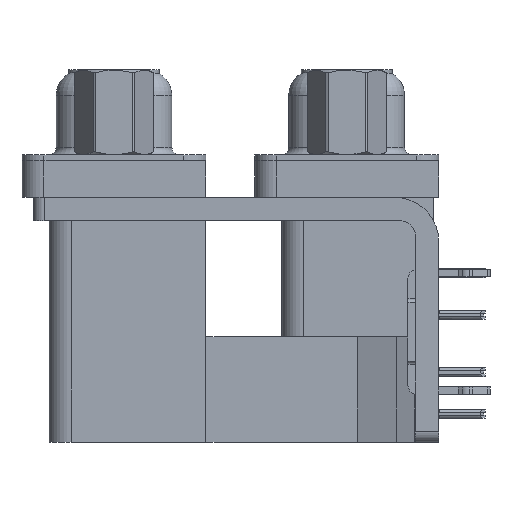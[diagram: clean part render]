
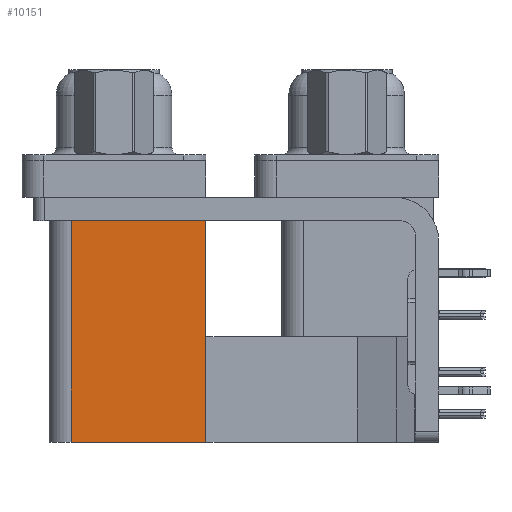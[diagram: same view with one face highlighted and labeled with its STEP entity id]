
A CAD part, left-side view. The second image highlights one B-rep face of the part: STEP entity #10151.
In plain terms, the highlighted planar face has unit normal (-1, 0, 0).
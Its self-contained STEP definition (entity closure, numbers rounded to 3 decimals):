
#3024 = EDGE_CURVE ( 'NONE', #4652, #26263, #17818, .T. ) ;
#3674 = AXIS2_PLACEMENT_3D ( 'NONE', #4900, #19683, #19929 ) ;
#4652 = VERTEX_POINT ( 'NONE', #45488 ) ;
#4900 = CARTESIAN_POINT ( 'NONE',  ( 3.79, 9.6, -19.2 ) ) ;
#7055 = DIRECTION ( 'NONE',  ( 0., 1., 0. ) ) ;
#7793 = CARTESIAN_POINT ( 'NONE',  ( 3.79, 18.8, -2.5 ) ) ;
#10151 = ADVANCED_FACE ( 'NONE', ( #31162 ), #35183, .F. ) ;
#10164 = VECTOR ( 'NONE', #33649, 1000. ) ;
#11570 = EDGE_CURVE ( 'NONE', #33424, #26263, #18388, .T. ) ;
#11729 = EDGE_CURVE ( 'NONE', #20270, #33424, #15848, .T. ) ;
#14652 = EDGE_CURVE ( 'NONE', #20270, #4652, #35381, .T. ) ;
#15076 = VECTOR ( 'NONE', #47637, 1000. ) ;
#15828 = ORIENTED_EDGE ( 'NONE', *, *, #14652, .T. ) ;
#15848 = LINE ( 'NONE', #42152, #46941 ) ;
#17818 = LINE ( 'NONE', #41332, #23950 ) ;
#18388 = LINE ( 'NONE', #41407, #10164 ) ;
#19683 = DIRECTION ( 'NONE',  ( 1., 0., 0. ) ) ;
#19929 = DIRECTION ( 'NONE',  ( 0., 1., 0. ) ) ;
#20270 = VERTEX_POINT ( 'NONE', #42374 ) ;
#23107 = ORIENTED_EDGE ( 'NONE', *, *, #11729, .F. ) ;
#23950 = VECTOR ( 'NONE', #7055, 1000. ) ;
#24110 = CARTESIAN_POINT ( 'NONE',  ( 3.79, 9.6, -19.2 ) ) ;
#24972 = ORIENTED_EDGE ( 'NONE', *, *, #11570, .F. ) ;
#26263 = VERTEX_POINT ( 'NONE', #7793 ) ;
#27074 = EDGE_LOOP ( 'NONE', ( #46487, #24972, #23107, #15828 ) ) ;
#30866 = CARTESIAN_POINT ( 'NONE',  ( 3.79, 18.8, -19.2 ) ) ;
#31162 = FACE_OUTER_BOUND ( 'NONE', #27074, .T. ) ;
#33424 = VERTEX_POINT ( 'NONE', #30866 ) ;
#33649 = DIRECTION ( 'NONE',  ( 0., 0., 1. ) ) ;
#35183 = PLANE ( 'NONE',  #3674 ) ;
#35381 = LINE ( 'NONE', #24110, #15076 ) ;
#39138 = DIRECTION ( 'NONE',  ( 0., 1., 0. ) ) ;
#41332 = CARTESIAN_POINT ( 'NONE',  ( 3.79, 9.6, -2.5 ) ) ;
#41407 = CARTESIAN_POINT ( 'NONE',  ( 3.79, 18.8, -19.2 ) ) ;
#42152 = CARTESIAN_POINT ( 'NONE',  ( 3.79, 9.6, -19.2 ) ) ;
#42374 = CARTESIAN_POINT ( 'NONE',  ( 3.79, 9.6, -19.2 ) ) ;
#45488 = CARTESIAN_POINT ( 'NONE',  ( 3.79, 9.6, -2.5 ) ) ;
#46487 = ORIENTED_EDGE ( 'NONE', *, *, #3024, .T. ) ;
#46941 = VECTOR ( 'NONE', #39138, 1000. ) ;
#47637 = DIRECTION ( 'NONE',  ( 0., 0., 1. ) ) ;
